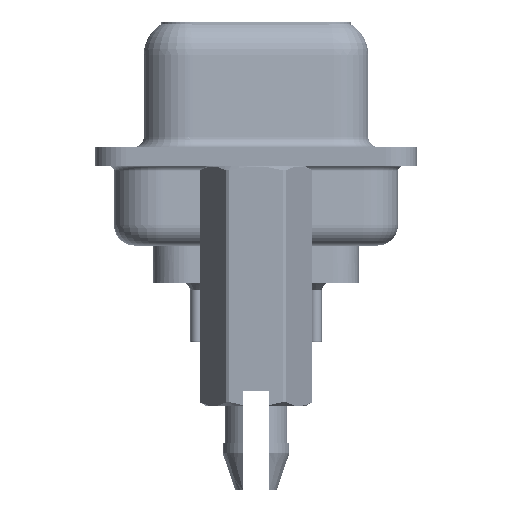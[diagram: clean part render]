
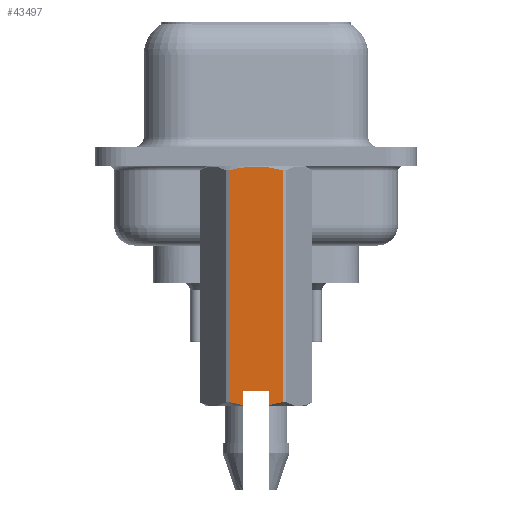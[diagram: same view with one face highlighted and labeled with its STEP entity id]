
A CAD part, left-side view. The second image highlights one B-rep face of the part: STEP entity #43497.
In plain terms, the highlighted planar face has unit normal (-1, 0, 0).
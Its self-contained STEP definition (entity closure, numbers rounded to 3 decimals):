
#26 = ORIENTED_EDGE ( 'NONE', *, *, #118, .F. ) ;
#118 = EDGE_CURVE ( 'NONE', #12055, #28532, #6293, .T. ) ;
#1437 = CARTESIAN_POINT ( 'NONE',  ( -2.381, -1.273, 0.581 ) ) ;
#1817 = LINE ( 'NONE', #1437, #14389 ) ;
#1836 = CARTESIAN_POINT ( 'NONE',  ( -2.381, 1.273, -11.748 ) ) ;
#2474 = PLANE ( 'NONE',  #4804 ) ;
#3067 = VERTEX_POINT ( 'NONE', #22484 ) ;
#3145 = CARTESIAN_POINT ( 'NONE',  ( -2.381, -1.273, -11.748 ) ) ;
#3324 = EDGE_CURVE ( 'NONE', #28532, #11280, #20539, .T. ) ;
#3537 = EDGE_CURVE ( 'NONE', #5011, #39206, #32905, .T. ) ;
#3750 = VERTEX_POINT ( 'NONE', #7588 ) ;
#4785 = EDGE_CURVE ( 'NONE', #12055, #3750, #6882, .T. ) ;
#4804 = AXIS2_PLACEMENT_3D ( 'NONE', #27084, #6325, #30527 ) ;
#5011 = VERTEX_POINT ( 'NONE', #21711 ) ;
#5341 = CARTESIAN_POINT ( 'NONE',  ( -2.381, 0.432, -0.485 ) ) ;
#5362 = B_SPLINE_CURVE_WITH_KNOTS ( 'NONE', 3,
 ( #17119, #20576, #30972, #10316 ),
 .UNSPECIFIED., .F., .F.,
 ( 4, 4 ),
 ( 0.003, 0.004 ),
 .UNSPECIFIED. ) ;
#5366 = CARTESIAN_POINT ( 'NONE',  ( -2.381, 0.625, -11.885 ) ) ;
#6293 = LINE ( 'NONE', #15722, #24758 ) ;
#6325 = DIRECTION ( 'NONE',  ( -1., 0., 0. ) ) ;
#6882 = LINE ( 'NONE', #16915, #33280 ) ;
#6958 = VERTEX_POINT ( 'NONE', #3145 ) ;
#7087 = ORIENTED_EDGE ( 'NONE', *, *, #18273, .T. ) ;
#7588 = CARTESIAN_POINT ( 'NONE',  ( -2.381, -0.625, -11.885 ) ) ;
#8502 = CARTESIAN_POINT ( 'NONE',  ( -2.381, -0.625, -11.2 ) ) ;
#8926 = CARTESIAN_POINT ( 'NONE',  ( -2.381, 1.066, -0.596 ) ) ;
#9296 = ORIENTED_EDGE ( 'NONE', *, *, #3537, .T. ) ;
#10316 = CARTESIAN_POINT ( 'NONE',  ( -2.381, -1.273, -11.748 ) ) ;
#10546 = EDGE_LOOP ( 'NONE', ( #42514, #26, #18550, #36113, #7087, #9296, #40925, #29292, #14197 ) ) ;
#10724 = CARTESIAN_POINT ( 'NONE',  ( -2.381, 0.845, -11.853 ) ) ;
#11280 = VERTEX_POINT ( 'NONE', #5366 ) ;
#11358 = VECTOR ( 'NONE', #18220, 1000. ) ;
#12055 = VERTEX_POINT ( 'NONE', #8502 ) ;
#13177 = EDGE_CURVE ( 'NONE', #3750, #6958, #5362, .T. ) ;
#14032 = CARTESIAN_POINT ( 'NONE',  ( -2.381, 1.273, -11.748 ) ) ;
#14197 = ORIENTED_EDGE ( 'NONE', *, *, #24768, .T. ) ;
#14285 = FACE_OUTER_BOUND ( 'NONE', #10546, .T. ) ;
#14389 = VECTOR ( 'NONE', #25743, 1000. ) ;
#15722 = CARTESIAN_POINT ( 'NONE',  ( -2.381, -0.625, -11.2 ) ) ;
#16915 = CARTESIAN_POINT ( 'NONE',  ( -2.381, -0.625, -11.2 ) ) ;
#16976 = DIRECTION ( 'NONE',  ( 0., 1., 0. ) ) ;
#17119 = CARTESIAN_POINT ( 'NONE',  ( -2.381, -0.625, -11.885 ) ) ;
#17522 = CARTESIAN_POINT ( 'NONE',  ( -2.381, 1.06, -11.806 ) ) ;
#18220 = DIRECTION ( 'NONE',  ( 0., 0., -1. ) ) ;
#18273 = EDGE_CURVE ( 'NONE', #6958, #5011, #1817, .T. ) ;
#18550 = ORIENTED_EDGE ( 'NONE', *, *, #4785, .T. ) ;
#20539 = LINE ( 'NONE', #32977, #11358 ) ;
#20576 = CARTESIAN_POINT ( 'NONE',  ( -2.381, -0.842, -11.854 ) ) ;
#21711 = CARTESIAN_POINT ( 'NONE',  ( -2.381, -1.273, -0.652 ) ) ;
#21733 = VECTOR ( 'NONE', #41605, 1000. ) ;
#22480 = VERTEX_POINT ( 'NONE', #1836 ) ;
#22484 = CARTESIAN_POINT ( 'NONE',  ( -2.381, 1.273, -0.652 ) ) ;
#24758 = VECTOR ( 'NONE', #16976, 1000. ) ;
#24768 = EDGE_CURVE ( 'NONE', #22480, #11280, #25532, .T. ) ;
#25532 = B_SPLINE_CURVE_WITH_KNOTS ( 'NONE', 3,
 ( #14032, #17522, #10724, #34725 ),
 .UNSPECIFIED., .F., .F.,
 ( 4, 4 ),
 ( 0.001, 0.002 ),
 .UNSPECIFIED. ) ;
#25743 = DIRECTION ( 'NONE',  ( 0., 0., 1. ) ) ;
#25978 = CARTESIAN_POINT ( 'NONE',  ( -2.381, 0.215, -0.468 ) ) ;
#26842 = EDGE_CURVE ( 'NONE', #3067, #22480, #30908, .T. ) ;
#27084 = CARTESIAN_POINT ( 'NONE',  ( -2.381, -1.375, -0.45 ) ) ;
#27336 = DIRECTION ( 'NONE',  ( 0., 0., -1. ) ) ;
#28011 = CARTESIAN_POINT ( 'NONE',  ( -2.381, 0.625, -11.2 ) ) ;
#28532 = VERTEX_POINT ( 'NONE', #28011 ) ;
#29292 = ORIENTED_EDGE ( 'NONE', *, *, #26842, .T. ) ;
#29573 = CARTESIAN_POINT ( 'NONE',  ( -2.381, 0.858, -0.55 ) ) ;
#30527 = DIRECTION ( 'NONE',  ( 0., 0., 1. ) ) ;
#30908 = LINE ( 'NONE', #31585, #21733 ) ;
#30972 = CARTESIAN_POINT ( 'NONE',  ( -2.381, -1.06, -11.806 ) ) ;
#31585 = CARTESIAN_POINT ( 'NONE',  ( -2.381, 1.273, 0.581 ) ) ;
#32905 = B_SPLINE_CURVE_WITH_KNOTS ( 'NONE', 3,
 ( #33762, #34295, #35205, #33710, #33607, #33465 ),
 .UNSPECIFIED., .F., .F.,
 ( 4, 2, 4 ),
 ( 0.003, 0.003, 0.004 ),
 .UNSPECIFIED. ) ;
#32962 = CARTESIAN_POINT ( 'NONE',  ( -2.381, 1.273, -0.652 ) ) ;
#32977 = CARTESIAN_POINT ( 'NONE',  ( -2.381, 0.625, -11.2 ) ) ;
#33280 = VECTOR ( 'NONE', #27336, 1000. ) ;
#33465 = CARTESIAN_POINT ( 'NONE',  ( -2.381, 0., -0.468 ) ) ;
#33607 = CARTESIAN_POINT ( 'NONE',  ( -2.381, -0.215, -0.468 ) ) ;
#33710 = CARTESIAN_POINT ( 'NONE',  ( -2.381, -0.428, -0.485 ) ) ;
#33762 = CARTESIAN_POINT ( 'NONE',  ( -2.381, -1.273, -0.652 ) ) ;
#34295 = CARTESIAN_POINT ( 'NONE',  ( -2.381, -1.065, -0.596 ) ) ;
#34725 = CARTESIAN_POINT ( 'NONE',  ( -2.381, 0.625, -11.885 ) ) ;
#35205 = CARTESIAN_POINT ( 'NONE',  ( -2.381, -0.853, -0.549 ) ) ;
#36113 = ORIENTED_EDGE ( 'NONE', *, *, #13177, .T. ) ;
#39206 = VERTEX_POINT ( 'NONE', #43225 ) ;
#40925 = ORIENTED_EDGE ( 'NONE', *, *, #41529, .T. ) ;
#41529 = EDGE_CURVE ( 'NONE', #39206, #3067, #43255, .T. ) ;
#41605 = DIRECTION ( 'NONE',  ( 0., 0., -1. ) ) ;
#42514 = ORIENTED_EDGE ( 'NONE', *, *, #3324, .F. ) ;
#43000 = CARTESIAN_POINT ( 'NONE',  ( -2.381, 0., -0.468 ) ) ;
#43225 = CARTESIAN_POINT ( 'NONE',  ( -2.381, 0., -0.468 ) ) ;
#43255 = B_SPLINE_CURVE_WITH_KNOTS ( 'NONE', 3,
 ( #43000, #25978, #5341, #29573, #8926, #32962 ),
 .UNSPECIFIED., .F., .F.,
 ( 4, 2, 4 ),
 ( 0.004, 0.004, 0.005 ),
 .UNSPECIFIED. ) ;
#43497 = ADVANCED_FACE ( 'NONE', ( #14285 ), #2474, .T. ) ;
